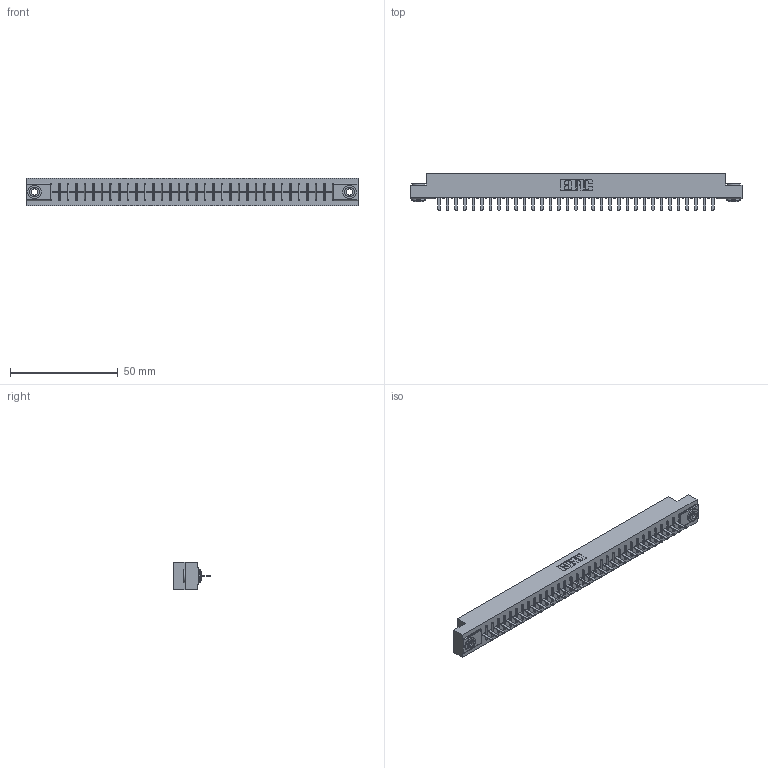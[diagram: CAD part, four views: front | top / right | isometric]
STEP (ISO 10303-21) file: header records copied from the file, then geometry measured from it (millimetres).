
FILE_DESCRIPTION (( 'STEP AP203' ), '1' );
FILE_NAME ('356-033-420-103.STEP', '2020-09-23T21:36:51', ( '' ), ( '' ), 'SwSTEP 2.0', 'SolidWorks 2020', '' );
FILE_SCHEMA (( 'CONFIG_CONTROL_DESIGN' ));
Length unit declared in the file: inch
Products named in the file (4): 306 Part_.156 Dia; 306-290-001_120; 356-033-420-103; 345-250-002_345-250-002-102
Assembly tree (36 placements, depth 2):
  356-033-420-103
    306 Part_.156 Dia
    306-290-001_120  x33
    345-250-002_345-250-002-102  x2
Bounding box: 153.77 x 17.12 x 12.7 mm (x, y, z)
Volume: 16927.3 mm3; surface area: 17549.5 mm2
Topology: 36 solids, 36 shells, 2478 faces, 6929 edges, 4438 vertices
Faces by surface type: plane 1643, cylinder 695, sphere 132, cone 8
Entity records: 32961 total; most frequent: CARTESIAN_POINT 5511, ORIENTED_EDGE 5454, DIRECTION 5449, EDGE_CURVE 2727, VECTOR 2121, LINE 2121, VERTEX_POINT 1726, AXIS2_PLACEMENT_3D 1664
